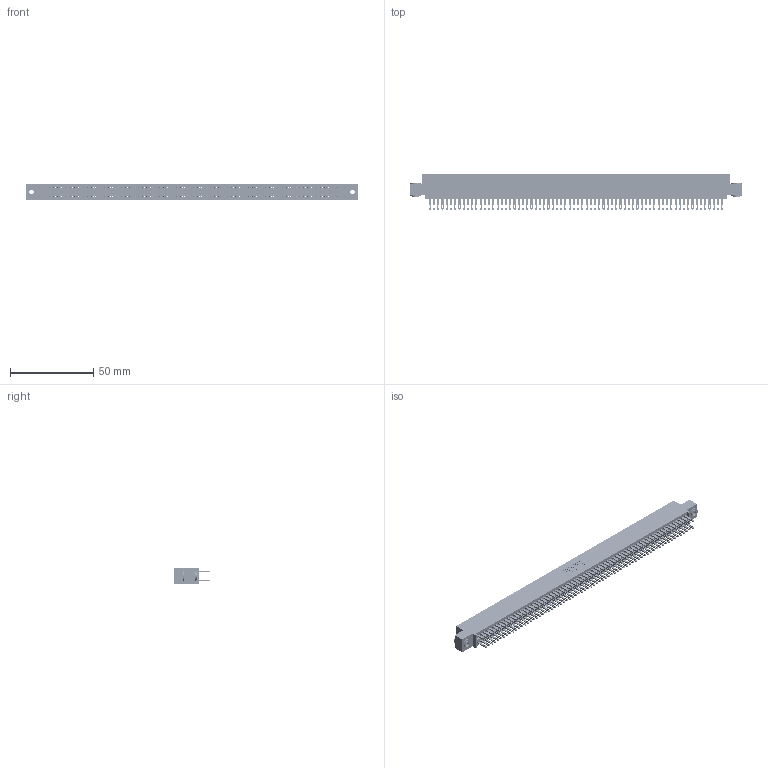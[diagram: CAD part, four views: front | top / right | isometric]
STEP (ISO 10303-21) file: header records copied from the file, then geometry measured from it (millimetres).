
FILE_DESCRIPTION (( 'STEP AP203' ), '1' );
FILE_NAME ('345-140-500-503.STEP', '2019-11-08T18:47:03', ( '' ), ( '' ), 'SwSTEP 2.0', 'SolidWorks 2016', '' );
FILE_SCHEMA (( 'CONFIG_CONTROL_DESIGN' ));
Length unit declared in the file: inch
Products named in the file (4): 345-140-500-503; 345-292-001_345-293-100; 345-250-002_345-250-002-102; 345 Part_0.110 Offset - 0.156 Dia-TH
Assembly tree (143 placements, depth 2):
  345-140-500-503
    345 Part_0.110 Offset - 0.156 Dia-TH
    345-292-001_345-293-100  x140
    345-250-002_345-250-002-102  x2
Bounding box: 199.01 x 21.51 x 9.4 mm (x, y, z)
Volume: 19965.7 mm3; surface area: 31780.6 mm2
Topology: 143 solids, 143 shells, 6608 faces, 20169 edges, 13442 vertices
Faces by surface type: plane 3874, cylinder 2726, cone 8
Entity records: 51866 total; most frequent: CARTESIAN_POINT 8643, ORIENTED_EDGE 8570, DIRECTION 7619, EDGE_CURVE 4285, LINE 3845, VECTOR 3845, VERTEX_POINT 2854, AXIS2_PLACEMENT_3D 1887
